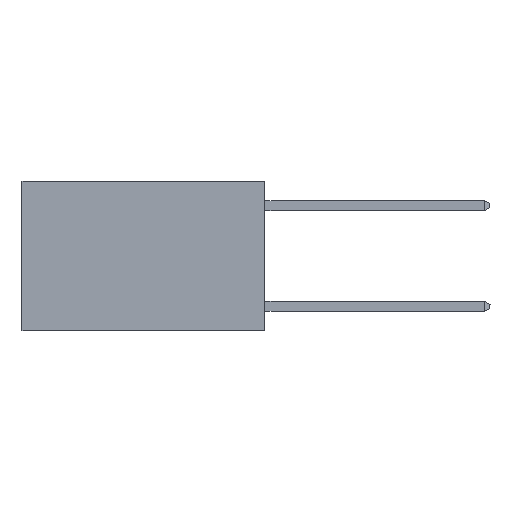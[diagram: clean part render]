
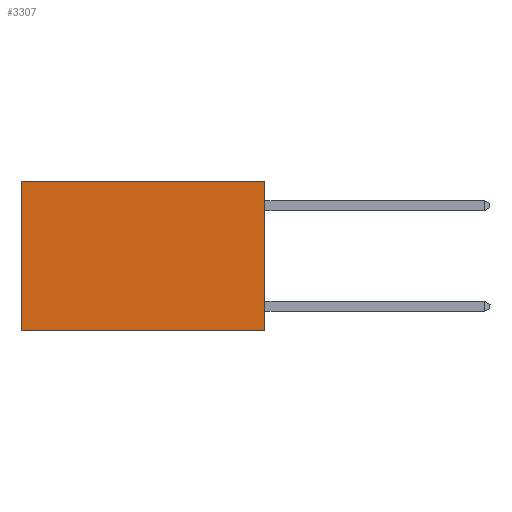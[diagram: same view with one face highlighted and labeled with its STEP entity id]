
A CAD part, left-side view. The second image highlights one B-rep face of the part: STEP entity #3307.
In plain terms, the highlighted planar face has unit normal (-1, 0, 0).
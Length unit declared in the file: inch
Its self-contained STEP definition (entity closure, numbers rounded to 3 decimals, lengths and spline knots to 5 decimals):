
#478 = VECTOR ( 'NONE', #26437, 39.37008 ) ;
#840 = VECTOR ( 'NONE', #11934, 39.37008 ) ;
#981 = LINE ( 'NONE', #16112, #8388 ) ;
#1398 = EDGE_CURVE ( 'NONE', #8068, #14770, #6322, .T. ) ;
#1492 = VECTOR ( 'NONE', #7352, 39.37008 ) ;
#1627 = PLANE ( 'NONE',  #5398 ) ;
#2053 = EDGE_CURVE ( 'NONE', #24339, #14770, #5972, .T. ) ;
#2474 = ORIENTED_EDGE ( 'NONE', *, *, #26305, .T. ) ;
#2881 = ORIENTED_EDGE ( 'NONE', *, *, #17836, .F. ) ;
#3118 = CARTESIAN_POINT ( 'NONE',  ( 0.2625, 0., 0. ) ) ;
#3307 = ADVANCED_FACE ( 'NONE', ( #8453 ), #1627, .F. ) ;
#3701 = CARTESIAN_POINT ( 'NONE',  ( 0.2625, 0., 0. ) ) ;
#4546 = CARTESIAN_POINT ( 'NONE',  ( 0.2625, 0., -0.37 ) ) ;
#4622 = CARTESIAN_POINT ( 'NONE',  ( 0.2625, 0., -0.37 ) ) ;
#5398 = AXIS2_PLACEMENT_3D ( 'NONE', #3701, #5791, #20249 ) ;
#5791 = DIRECTION ( 'NONE',  ( 1., 0., 0. ) ) ;
#5972 = LINE ( 'NONE', #25565, #478 ) ;
#6322 = LINE ( 'NONE', #4622, #840 ) ;
#7188 = CARTESIAN_POINT ( 'NONE',  ( 0.2625, 0.6, 0. ) ) ;
#7352 = DIRECTION ( 'NONE',  ( 0., 0., -1. ) ) ;
#7825 = DIRECTION ( 'NONE',  ( 0., 1., 0. ) ) ;
#7877 = EDGE_LOOP ( 'NONE', ( #8959, #13589, #2881, #2474 ) ) ;
#8068 = VERTEX_POINT ( 'NONE', #4546 ) ;
#8388 = VECTOR ( 'NONE', #7825, 39.37008 ) ;
#8453 = FACE_OUTER_BOUND ( 'NONE', #7877, .T. ) ;
#8959 = ORIENTED_EDGE ( 'NONE', *, *, #2053, .T. ) ;
#11070 = CARTESIAN_POINT ( 'NONE',  ( 0.2625, 0., 0. ) ) ;
#11670 = VERTEX_POINT ( 'NONE', #11070 ) ;
#11934 = DIRECTION ( 'NONE',  ( 0., 1., 0. ) ) ;
#13589 = ORIENTED_EDGE ( 'NONE', *, *, #1398, .F. ) ;
#14770 = VERTEX_POINT ( 'NONE', #16491 ) ;
#16112 = CARTESIAN_POINT ( 'NONE',  ( 0.2625, 0., 0. ) ) ;
#16491 = CARTESIAN_POINT ( 'NONE',  ( 0.2625, 0.6, -0.37 ) ) ;
#17836 = EDGE_CURVE ( 'NONE', #11670, #8068, #23435, .T. ) ;
#20249 = DIRECTION ( 'NONE',  ( 0., 0., -1. ) ) ;
#23435 = LINE ( 'NONE', #3118, #1492 ) ;
#24339 = VERTEX_POINT ( 'NONE', #7188 ) ;
#25565 = CARTESIAN_POINT ( 'NONE',  ( 0.2625, 0.6, 0. ) ) ;
#26305 = EDGE_CURVE ( 'NONE', #11670, #24339, #981, .T. ) ;
#26437 = DIRECTION ( 'NONE',  ( 0., 0., -1. ) ) ;
